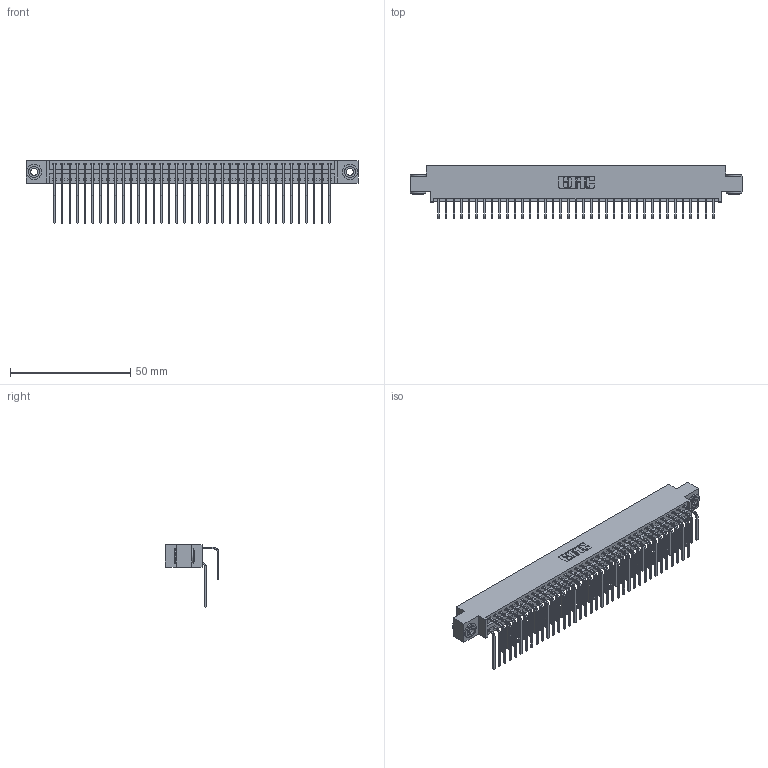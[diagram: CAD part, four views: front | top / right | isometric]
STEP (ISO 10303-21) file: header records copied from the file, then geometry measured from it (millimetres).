
FILE_DESCRIPTION (( 'STEP AP203' ), '1' );
FILE_NAME ('396-074-558-803.STEP', '2019-11-03T11:43:09', ( '' ), ( '' ), 'SwSTEP 2.0', 'SolidWorks 2016', '' );
FILE_SCHEMA (( 'CONFIG_CONTROL_DESIGN' ));
Length unit declared in the file: inch
Products named in the file (5): 345-292-001_558 Tail - 2; 345-250-002_345-250-002-102; 345-292-001_558 559 Tail - 1; 396-074-558-803; 346 Part_0.170 Offset - 0.156 Dia-TH
Assembly tree (77 placements, depth 2):
  396-074-558-803
    346 Part_0.170 Offset - 0.156 Dia-TH
    345-292-001_558 559 Tail - 1  x37
    345-292-001_558 Tail - 2  x37
    345-250-002_345-250-002-102  x2
Bounding box: 138.05 x 22.16 x 26.16 mm (x, y, z)
Volume: 13714.3 mm3; surface area: 21214.4 mm2
Topology: 77 solids, 77 shells, 4160 faces, 12331 edges, 8118 vertices
Faces by surface type: plane 2828, cylinder 1324, cone 8
Entity records: 27386 total; most frequent: CARTESIAN_POINT 4550, ORIENTED_EDGE 4426, DIRECTION 4063, EDGE_CURVE 2213, VECTOR 1869, LINE 1869, VERTEX_POINT 1470, AXIS2_PLACEMENT_3D 1097
